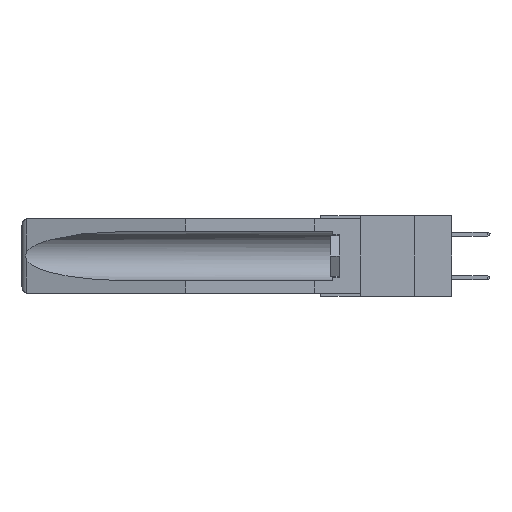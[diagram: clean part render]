
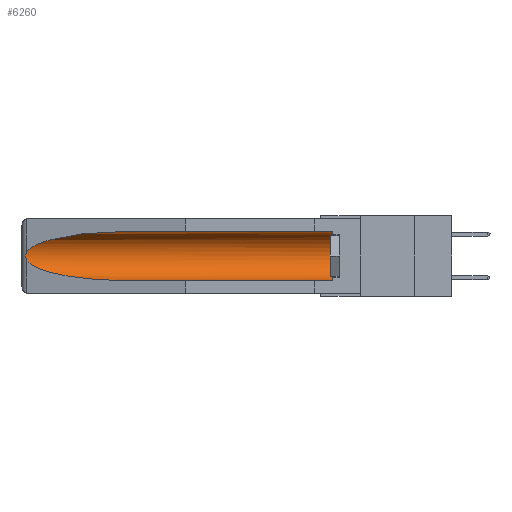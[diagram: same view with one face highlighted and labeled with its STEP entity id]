
A CAD part, left-side view. The second image highlights one B-rep face of the part: STEP entity #6260.
In plain terms, the highlighted cylindrical face has radius 2.857 mm (diameter 5.715 mm), a partial arc.
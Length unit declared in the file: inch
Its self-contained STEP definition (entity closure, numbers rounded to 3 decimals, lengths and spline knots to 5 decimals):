
#23 = DIRECTION ( 'NONE',  ( 0., 1., 0. ) ) ;
#358 = CARTESIAN_POINT ( 'NONE',  ( 0.26597, 1.52961, -0.15275 ) ) ;
#771 = CARTESIAN_POINT ( 'NONE',  ( 0.155, 1.07973, -0.284 ) ) ;
#928 = B_SPLINE_CURVE_WITH_KNOTS ( 'NONE', 3,
 ( #15933, #358, #2915, #25635, #28596, #18127, #13068, #5490, #20522, #3024 ),
 .UNSPECIFIED., .F., .F.,
 ( 4, 2, 2, 2, 4 ),
 ( 0., 0.00029, 0.00058, 0.00087, 0.00117 ),
 .UNSPECIFIED. ) ;
#1271 = CARTESIAN_POINT ( 'NONE',  ( 0.26537, 1.52718, -0.19328 ) ) ;
#1423 = CARTESIAN_POINT ( 'NONE',  ( 0.155, 1.07973, -0.059 ) ) ;
#2134 = EDGE_CURVE ( 'NONE', #6983, #32288, #17115, .T. ) ;
#2915 = CARTESIAN_POINT ( 'NONE',  ( 0.26654, 1.53092, -0.15636 ) ) ;
#3024 = CARTESIAN_POINT ( 'NONE',  ( 0.26537, 1.52718, -0.19328 ) ) ;
#3764 = CARTESIAN_POINT ( 'NONE',  ( 0.26537, 1.52718, -0.14972 ) ) ;
#4512 = VECTOR ( 'NONE', #24473, 39.37008 ) ;
#5347 = CARTESIAN_POINT ( 'NONE',  ( 0.25451, 1.48313, -0.24835 ) ) ;
#5490 = CARTESIAN_POINT ( 'NONE',  ( 0.26655, 1.53094, -0.18657 ) ) ;
#6260 = ADVANCED_FACE ( 'NONE', ( #12368 ), #6529, .F. ) ;
#6529 = CYLINDRICAL_SURFACE ( 'NONE', #10985, 0.1125 ) ;
#6983 = VERTEX_POINT ( 'NONE', #13114 ) ;
#8593 = DIRECTION ( 'NONE',  ( 0., 0., 1. ) ) ;
#8981 = CARTESIAN_POINT ( 'NONE',  ( 0.21114, 1.30732, -0.059 ) ) ;
#9002 = ORIENTED_EDGE ( 'NONE', *, *, #23097, .F. ) ;
#9630 = CARTESIAN_POINT ( 'NONE',  ( 0.155, -0.30754, -0.284 ) ) ;
#10386 = ORIENTED_EDGE ( 'NONE', *, *, #26412, .T. ) ;
#10406 = CARTESIAN_POINT ( 'NONE',  ( 0.21114, 1.30732, -0.284 ) ) ;
#10689 = CARTESIAN_POINT ( 'NONE',  ( 0.26537, 1.52718, -0.14972 ) ) ;
#10985 = AXIS2_PLACEMENT_3D ( 'NONE', #13664, #26001, #23883 ) ;
#11805 = ORIENTED_EDGE ( 'NONE', *, *, #17886, .T. ) ;
#12350 = VERTEX_POINT ( 'NONE', #13978 ) ;
#12368 = FACE_OUTER_BOUND ( 'NONE', #29720, .T. ) ;
#12964 = VERTEX_POINT ( 'NONE', #21382 ) ;
#13068 = CARTESIAN_POINT ( 'NONE',  ( 0.2673, 1.53269, -0.17917 ) ) ;
#13114 = CARTESIAN_POINT ( 'NONE',  ( 0.155, 1.07973, -0.059 ) ) ;
#13511 = ORIENTED_EDGE ( 'NONE', *, *, #2134, .T. ) ;
#13664 = CARTESIAN_POINT ( 'NONE',  ( 0.155, -0.30754, -0.1715 ) ) ;
#13767 = CARTESIAN_POINT ( 'NONE',  ( 0.155, 0.126, -0.284 ) ) ;
#13978 = CARTESIAN_POINT ( 'NONE',  ( 0.155, 0.126, -0.059 ) ) ;
#14158 = ORIENTED_EDGE ( 'NONE', *, *, #17371, .T. ) ;
#15094 = VERTEX_POINT ( 'NONE', #13767 ) ;
#15933 = CARTESIAN_POINT ( 'NONE',  ( 0.26537, 1.52718, -0.14972 ) ) ;
#16482 = VERTEX_POINT ( 'NONE', #771 ) ;
#17115 =( BOUNDED_CURVE ( )  B_SPLINE_CURVE ( 3, ( #1423, #8981, #31638, #3764 ),
 .UNSPECIFIED., .F., .F. ) 
 B_SPLINE_CURVE_WITH_KNOTS ( ( 4, 4 ),
 ( 4.71239, 6.08839 ),
 .UNSPECIFIED. ) 
 CURVE ( )  GEOMETRIC_REPRESENTATION_ITEM ( )  RATIONAL_B_SPLINE_CURVE ( ( 1., 0.848, 0.848, 1. ) ) 
 REPRESENTATION_ITEM ( '' )  );
#17371 = EDGE_CURVE ( 'NONE', #32288, #12964, #928, .T. ) ;
#17886 = EDGE_CURVE ( 'NONE', #12964, #16482, #18121, .T. ) ;
#18121 =( BOUNDED_CURVE ( )  B_SPLINE_CURVE ( 3, ( #1271, #5347, #10406, #23239 ),
 .UNSPECIFIED., .F., .F. ) 
 B_SPLINE_CURVE_WITH_KNOTS ( ( 4, 4 ),
 ( 0.1948, 1.5708 ),
 .UNSPECIFIED. ) 
 CURVE ( )  GEOMETRIC_REPRESENTATION_ITEM ( )  RATIONAL_B_SPLINE_CURVE ( ( 1., 0.848, 0.848, 1. ) ) 
 REPRESENTATION_ITEM ( '' )  );
#18127 = CARTESIAN_POINT ( 'NONE',  ( 0.2675, 1.53308, -0.17534 ) ) ;
#20522 = CARTESIAN_POINT ( 'NONE',  ( 0.26597, 1.5296, -0.19026 ) ) ;
#20696 = EDGE_CURVE ( 'NONE', #15094, #12350, #27162, .T. ) ;
#21065 = DIRECTION ( 'NONE',  ( 0., -1., 0. ) ) ;
#21382 = CARTESIAN_POINT ( 'NONE',  ( 0.26537, 1.52718, -0.19328 ) ) ;
#23097 = EDGE_CURVE ( 'NONE', #15094, #16482, #32084, .T. ) ;
#23239 = CARTESIAN_POINT ( 'NONE',  ( 0.155, 1.07973, -0.284 ) ) ;
#23883 = DIRECTION ( 'NONE',  ( 0., 0., 1. ) ) ;
#24350 = ORIENTED_EDGE ( 'NONE', *, *, #20696, .T. ) ;
#24473 = DIRECTION ( 'NONE',  ( 0., 1., 0. ) ) ;
#25635 = CARTESIAN_POINT ( 'NONE',  ( 0.2673, 1.5327, -0.16383 ) ) ;
#26001 = DIRECTION ( 'NONE',  ( 0., 1., 0. ) ) ;
#26412 = EDGE_CURVE ( 'NONE', #12350, #6983, #27914, .T. ) ;
#26909 = AXIS2_PLACEMENT_3D ( 'NONE', #29051, #21065, #8593 ) ;
#27162 = CIRCLE ( 'NONE', #26909, 0.1125 ) ;
#27730 = CARTESIAN_POINT ( 'NONE',  ( 0.155, -0.30754, -0.059 ) ) ;
#27914 = LINE ( 'NONE', #27730, #31055 ) ;
#28596 = CARTESIAN_POINT ( 'NONE',  ( 0.2675, 1.53308, -0.16763 ) ) ;
#29051 = CARTESIAN_POINT ( 'NONE',  ( 0.155, 0.126, -0.1715 ) ) ;
#29720 = EDGE_LOOP ( 'NONE', ( #13511, #14158, #11805, #9002, #24350, #10386 ) ) ;
#31055 = VECTOR ( 'NONE', #23, 39.37008 ) ;
#31638 = CARTESIAN_POINT ( 'NONE',  ( 0.25451, 1.48313, -0.09465 ) ) ;
#32084 = LINE ( 'NONE', #9630, #4512 ) ;
#32288 = VERTEX_POINT ( 'NONE', #10689 ) ;
